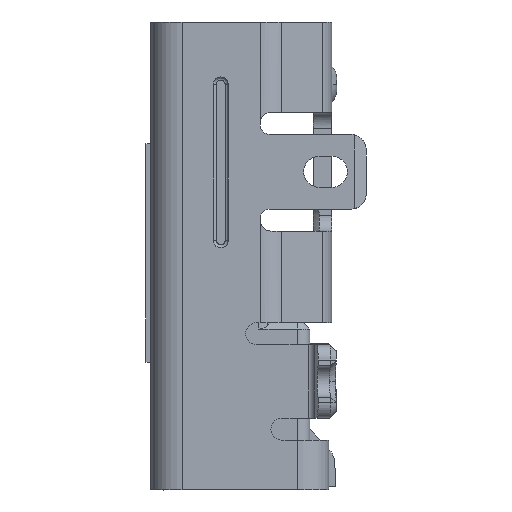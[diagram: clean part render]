
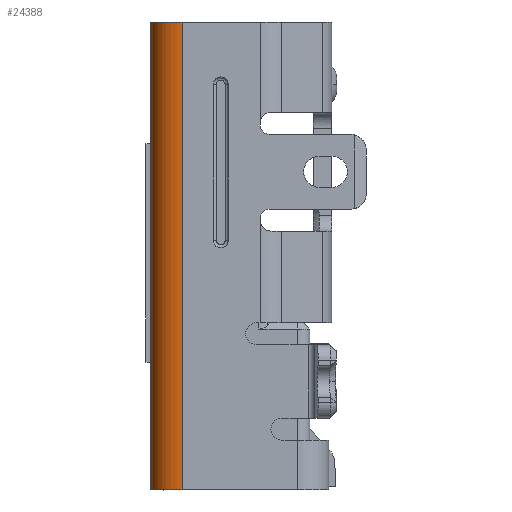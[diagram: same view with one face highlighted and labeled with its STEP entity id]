
A CAD part, left-side view. The second image highlights one B-rep face of the part: STEP entity #24388.
In plain terms, the highlighted cylindrical face has radius 0.5 mm (diameter 1 mm), a partial arc.
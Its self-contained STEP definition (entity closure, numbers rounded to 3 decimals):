
#2541 = CYLINDRICAL_SURFACE ( 'NONE', #22214, 0.5 ) ;
#6512 = ORIENTED_EDGE ( 'NONE', *, *, #52390, .F. ) ;
#8971 = VERTEX_POINT ( 'NONE', #9684 ) ;
#9684 = CARTESIAN_POINT ( 'NONE',  ( -2.75, 0., 0. ) ) ;
#11807 = EDGE_LOOP ( 'NONE', ( #54196, #33280, #6512, #31286 ) ) ;
#12649 = VERTEX_POINT ( 'NONE', #21963 ) ;
#12928 = FACE_OUTER_BOUND ( 'NONE', #11807, .T. ) ;
#12986 = CARTESIAN_POINT ( 'NONE',  ( -3.25, -0.5, -3.75 ) ) ;
#14041 = VECTOR ( 'NONE', #60382, 1000. ) ;
#14345 = CARTESIAN_POINT ( 'NONE',  ( -2.75, -0.5, 0. ) ) ;
#17747 = AXIS2_PLACEMENT_3D ( 'NONE', #33907, #38133, #58058 ) ;
#18282 = VERTEX_POINT ( 'NONE', #28181 ) ;
#21963 = CARTESIAN_POINT ( 'NONE',  ( -3.25, -0.5, 0. ) ) ;
#22214 = AXIS2_PLACEMENT_3D ( 'NONE', #47468, #57009, #47156 ) ;
#22799 = LINE ( 'NONE', #12986, #30486 ) ;
#23787 = DIRECTION ( 'NONE',  ( -1., 0., 0. ) ) ;
#24388 = ADVANCED_FACE ( 'NONE', ( #12928 ), #2541, .T. ) ;
#24434 = DIRECTION ( 'NONE',  ( 0., 0., 1. ) ) ;
#28181 = CARTESIAN_POINT ( 'NONE',  ( -3.25, -0.5, -7.5 ) ) ;
#29878 = AXIS2_PLACEMENT_3D ( 'NONE', #14345, #24434, #23787 ) ;
#30486 = VECTOR ( 'NONE', #42663, 1000. ) ;
#31286 = ORIENTED_EDGE ( 'NONE', *, *, #63659, .F. ) ;
#33280 = ORIENTED_EDGE ( 'NONE', *, *, #59398, .F. ) ;
#33907 = CARTESIAN_POINT ( 'NONE',  ( -2.75, -0.5, -7.5 ) ) ;
#35253 = CARTESIAN_POINT ( 'NONE',  ( -2.75, 0., 0.15 ) ) ;
#38133 = DIRECTION ( 'NONE',  ( 0., 0., -1. ) ) ;
#39665 = CIRCLE ( 'NONE', #17747, 0.5 ) ;
#42663 = DIRECTION ( 'NONE',  ( 0., 0., -1. ) ) ;
#44268 = EDGE_CURVE ( 'NONE', #45874, #8971, #45971, .T. ) ;
#45874 = VERTEX_POINT ( 'NONE', #48955 ) ;
#45971 = LINE ( 'NONE', #35253, #14041 ) ;
#47156 = DIRECTION ( 'NONE',  ( -1., 0., 0. ) ) ;
#47468 = CARTESIAN_POINT ( 'NONE',  ( -2.75, -0.5, 0. ) ) ;
#48955 = CARTESIAN_POINT ( 'NONE',  ( -2.75, 0., -7.5 ) ) ;
#52390 = EDGE_CURVE ( 'NONE', #12649, #18282, #22799, .T. ) ;
#54196 = ORIENTED_EDGE ( 'NONE', *, *, #44268, .F. ) ;
#57009 = DIRECTION ( 'NONE',  ( 0., 0., -1. ) ) ;
#57968 = CIRCLE ( 'NONE', #29878, 0.5 ) ;
#58058 = DIRECTION ( 'NONE',  ( -1., 0., 0. ) ) ;
#59398 = EDGE_CURVE ( 'NONE', #18282, #45874, #39665, .T. ) ;
#60382 = DIRECTION ( 'NONE',  ( 0., 0., 1. ) ) ;
#63659 = EDGE_CURVE ( 'NONE', #8971, #12649, #57968, .T. ) ;
